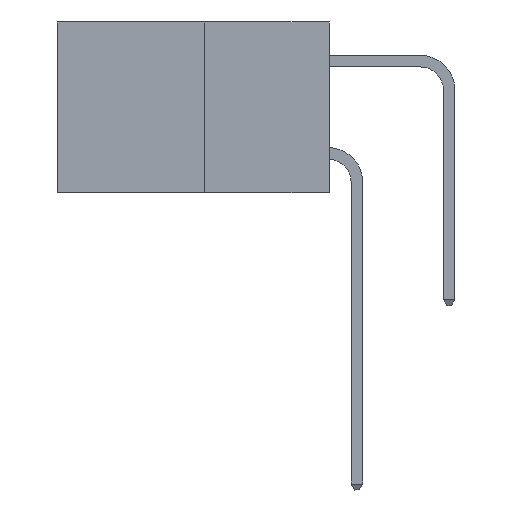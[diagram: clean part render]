
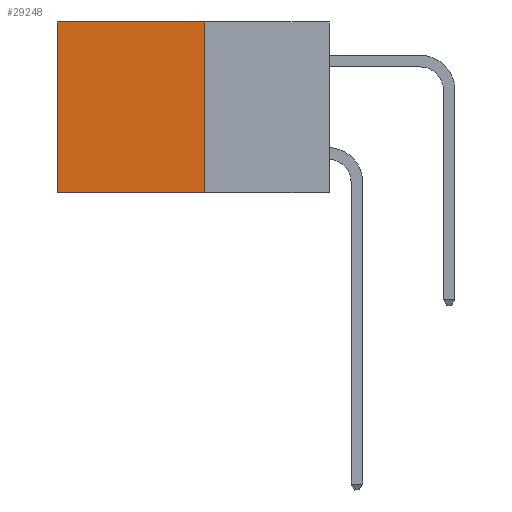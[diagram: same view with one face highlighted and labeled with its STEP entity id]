
A CAD part, left-side view. The second image highlights one B-rep face of the part: STEP entity #29248.
In plain terms, the highlighted planar face has unit normal (-1, 0, 0).
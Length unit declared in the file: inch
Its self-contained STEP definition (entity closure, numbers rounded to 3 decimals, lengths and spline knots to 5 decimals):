
#466 = ORIENTED_EDGE ( 'NONE', *, *, #29768, .F. ) ;
#2366 = VERTEX_POINT ( 'NONE', #28242 ) ;
#2687 = LINE ( 'NONE', #32887, #34062 ) ;
#4834 = DIRECTION ( 'NONE',  ( 0., 1., 0. ) ) ;
#5301 = LINE ( 'NONE', #32308, #19577 ) ;
#6487 = VERTEX_POINT ( 'NONE', #19242 ) ;
#7309 = AXIS2_PLACEMENT_3D ( 'NONE', #28525, #14167, #34275 ) ;
#8480 = EDGE_LOOP ( 'NONE', ( #20343, #466, #19870, #21469 ) ) ;
#8740 = LINE ( 'NONE', #24829, #16323 ) ;
#9304 = DIRECTION ( 'NONE',  ( 0., 0., -1. ) ) ;
#9979 = VERTEX_POINT ( 'NONE', #26272 ) ;
#11316 = PLANE ( 'NONE',  #7309 ) ;
#11800 = EDGE_CURVE ( 'NONE', #28740, #9979, #23608, .T. ) ;
#14167 = DIRECTION ( 'NONE',  ( 1., 0., 0. ) ) ;
#15627 = DIRECTION ( 'NONE',  ( 0., 1., 0. ) ) ;
#16262 = CARTESIAN_POINT ( 'NONE',  ( 0.277, 0.27, 0. ) ) ;
#16323 = VECTOR ( 'NONE', #4834, 39.37008 ) ;
#19242 = CARTESIAN_POINT ( 'NONE',  ( 0.277, 0.59, -0.37 ) ) ;
#19577 = VECTOR ( 'NONE', #9304, 39.37008 ) ;
#19870 = ORIENTED_EDGE ( 'NONE', *, *, #11800, .F. ) ;
#20343 = ORIENTED_EDGE ( 'NONE', *, *, #34924, .T. ) ;
#21469 = ORIENTED_EDGE ( 'NONE', *, *, #33675, .T. ) ;
#22611 = CARTESIAN_POINT ( 'NONE',  ( 0.277, 0.27, -0.37 ) ) ;
#23608 = LINE ( 'NONE', #22611, #30366 ) ;
#24829 = CARTESIAN_POINT ( 'NONE',  ( 0.277, 0.27, -0.37 ) ) ;
#26272 = CARTESIAN_POINT ( 'NONE',  ( 0.277, 0.27, -0.37 ) ) ;
#28242 = CARTESIAN_POINT ( 'NONE',  ( 0.277, 0.59, 0. ) ) ;
#28525 = CARTESIAN_POINT ( 'NONE',  ( 0.277, 0.27, -0.37 ) ) ;
#28740 = VERTEX_POINT ( 'NONE', #16262 ) ;
#29248 = ADVANCED_FACE ( 'NONE', ( #32607 ), #11316, .F. ) ;
#29768 = EDGE_CURVE ( 'NONE', #9979, #6487, #8740, .T. ) ;
#30366 = VECTOR ( 'NONE', #37027, 39.37008 ) ;
#32308 = CARTESIAN_POINT ( 'NONE',  ( 0.277, 0.59, -0.37 ) ) ;
#32607 = FACE_OUTER_BOUND ( 'NONE', #8480, .T. ) ;
#32887 = CARTESIAN_POINT ( 'NONE',  ( 0.277, 0.27, 0. ) ) ;
#33675 = EDGE_CURVE ( 'NONE', #28740, #2366, #2687, .T. ) ;
#34062 = VECTOR ( 'NONE', #15627, 39.37008 ) ;
#34275 = DIRECTION ( 'NONE',  ( 0., 0., -1. ) ) ;
#34924 = EDGE_CURVE ( 'NONE', #2366, #6487, #5301, .T. ) ;
#37027 = DIRECTION ( 'NONE',  ( 0., 0., -1. ) ) ;
